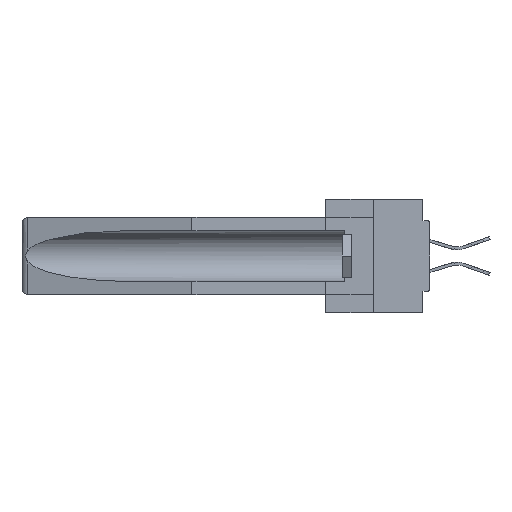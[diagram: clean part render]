
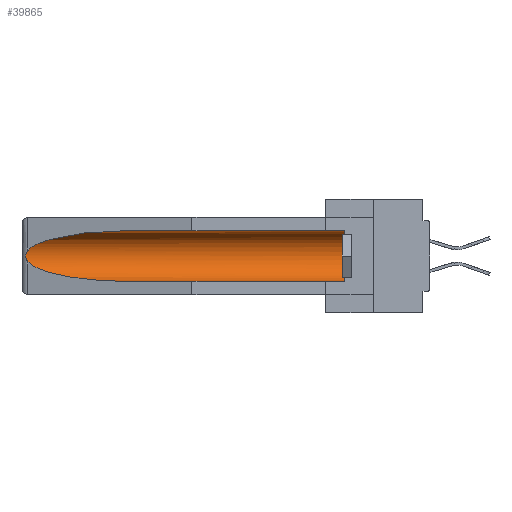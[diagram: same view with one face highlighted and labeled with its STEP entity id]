
A CAD part, left-side view. The second image highlights one B-rep face of the part: STEP entity #39865.
In plain terms, the highlighted cylindrical face has radius 2.857 mm (diameter 5.715 mm), a partial arc.
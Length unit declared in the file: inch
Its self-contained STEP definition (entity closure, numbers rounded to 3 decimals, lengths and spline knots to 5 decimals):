
#250 = B_SPLINE_CURVE_WITH_KNOTS ( 'NONE', 3,
 ( #32908, #36458, #30248, #26725, #6986, #30392, #23396, #7128, #13516, #16598 ),
 .UNSPECIFIED., .F., .F.,
 ( 4, 2, 2, 2, 4 ),
 ( 0., 0.00029, 0.00058, 0.00087, 0.00117 ),
 .UNSPECIFIED. ) ;
#292 = CYLINDRICAL_SURFACE ( 'NONE', #24004, 0.1125 ) ;
#764 = CARTESIAN_POINT ( 'NONE',  ( 0.155, 0.126, -0.284 ) ) ;
#2625 = VECTOR ( 'NONE', #35046, 39.37008 ) ;
#2854 = DIRECTION ( 'NONE',  ( 0., 1., 0. ) ) ;
#3840 = EDGE_CURVE ( 'NONE', #23100, #32858, #10617, .T. ) ;
#4747 = CARTESIAN_POINT ( 'NONE',  ( 0.26537, 1.52718, -0.19328 ) ) ;
#6986 = CARTESIAN_POINT ( 'NONE',  ( 0.2675, 1.53308, -0.16763 ) ) ;
#7058 = CARTESIAN_POINT ( 'NONE',  ( 0.21114, 1.30732, -0.284 ) ) ;
#7128 = CARTESIAN_POINT ( 'NONE',  ( 0.26655, 1.53094, -0.18657 ) ) ;
#7824 = CIRCLE ( 'NONE', #17391, 0.1125 ) ;
#8204 = VECTOR ( 'NONE', #8627, 39.37008 ) ;
#8316 = CARTESIAN_POINT ( 'NONE',  ( 0.155, -0.30754, -0.059 ) ) ;
#8610 = EDGE_CURVE ( 'NONE', #11835, #23100, #250, .T. ) ;
#8627 = DIRECTION ( 'NONE',  ( 0., 1., 0. ) ) ;
#9091 = CARTESIAN_POINT ( 'NONE',  ( 0.21114, 1.30732, -0.059 ) ) ;
#9203 = DIRECTION ( 'NONE',  ( 0., -1., 0. ) ) ;
#10617 =( BOUNDED_CURVE ( )  B_SPLINE_CURVE ( 3, ( #14150, #40654, #7058, #34012 ),
 .UNSPECIFIED., .F., .T. ) 
 B_SPLINE_CURVE_WITH_KNOTS ( ( 4, 4 ),
 ( 0.1948, 1.5708 ),
 .UNSPECIFIED. ) 
 CURVE ( )  GEOMETRIC_REPRESENTATION_ITEM ( )  RATIONAL_B_SPLINE_CURVE ( ( 1., 0.848, 0.848, 1. ) ) 
 REPRESENTATION_ITEM ( '' )  );
#11644 = LINE ( 'NONE', #25319, #2625 ) ;
#11835 = VERTEX_POINT ( 'NONE', #36188 ) ;
#13516 = CARTESIAN_POINT ( 'NONE',  ( 0.26597, 1.5296, -0.19026 ) ) ;
#14150 = CARTESIAN_POINT ( 'NONE',  ( 0.26537, 1.52718, -0.19328 ) ) ;
#15276 = CARTESIAN_POINT ( 'NONE',  ( 0.155, 0.126, -0.059 ) ) ;
#16598 = CARTESIAN_POINT ( 'NONE',  ( 0.26537, 1.52718, -0.19328 ) ) ;
#17274 = ORIENTED_EDGE ( 'NONE', *, *, #36701, .T. ) ;
#17391 = AXIS2_PLACEMENT_3D ( 'NONE', #19543, #9203, #18646 ) ;
#18308 = EDGE_LOOP ( 'NONE', ( #17274, #29156, #29476, #43070, #39761, #18794 ) ) ;
#18436 =( BOUNDED_CURVE ( )  B_SPLINE_CURVE ( 3, ( #19293, #9091, #39552, #19436 ),
 .UNSPECIFIED., .F., .F. ) 
 B_SPLINE_CURVE_WITH_KNOTS ( ( 4, 4 ),
 ( 4.71239, 6.08839 ),
 .UNSPECIFIED. ) 
 CURVE ( )  GEOMETRIC_REPRESENTATION_ITEM ( )  RATIONAL_B_SPLINE_CURVE ( ( 1., 0.848, 0.848, 1. ) ) 
 REPRESENTATION_ITEM ( '' )  );
#18646 = DIRECTION ( 'NONE',  ( 0., 0., 1. ) ) ;
#18794 = ORIENTED_EDGE ( 'NONE', *, *, #40266, .T. ) ;
#19293 = CARTESIAN_POINT ( 'NONE',  ( 0.155, 1.07973, -0.059 ) ) ;
#19436 = CARTESIAN_POINT ( 'NONE',  ( 0.26537, 1.52718, -0.14972 ) ) ;
#19543 = CARTESIAN_POINT ( 'NONE',  ( 0.155, 0.126, -0.1715 ) ) ;
#20162 = EDGE_CURVE ( 'NONE', #38524, #30199, #7824, .T. ) ;
#20185 = CARTESIAN_POINT ( 'NONE',  ( 0.155, -0.30754, -0.1715 ) ) ;
#23100 = VERTEX_POINT ( 'NONE', #4747 ) ;
#23396 = CARTESIAN_POINT ( 'NONE',  ( 0.2673, 1.53269, -0.17917 ) ) ;
#23558 = DIRECTION ( 'NONE',  ( 0., 0., 1. ) ) ;
#24004 = AXIS2_PLACEMENT_3D ( 'NONE', #20185, #2854, #23558 ) ;
#25319 = CARTESIAN_POINT ( 'NONE',  ( 0.155, -0.30754, -0.284 ) ) ;
#26725 = CARTESIAN_POINT ( 'NONE',  ( 0.2673, 1.5327, -0.16383 ) ) ;
#29156 = ORIENTED_EDGE ( 'NONE', *, *, #8610, .T. ) ;
#29476 = ORIENTED_EDGE ( 'NONE', *, *, #3840, .T. ) ;
#30199 = VERTEX_POINT ( 'NONE', #15276 ) ;
#30248 = CARTESIAN_POINT ( 'NONE',  ( 0.26654, 1.53092, -0.15636 ) ) ;
#30392 = CARTESIAN_POINT ( 'NONE',  ( 0.2675, 1.53308, -0.17534 ) ) ;
#32858 = VERTEX_POINT ( 'NONE', #36733 ) ;
#32908 = CARTESIAN_POINT ( 'NONE',  ( 0.26537, 1.52718, -0.14972 ) ) ;
#33502 = LINE ( 'NONE', #8316, #8204 ) ;
#34012 = CARTESIAN_POINT ( 'NONE',  ( 0.155, 1.07973, -0.284 ) ) ;
#34392 = EDGE_CURVE ( 'NONE', #38524, #32858, #11644, .T. ) ;
#35046 = DIRECTION ( 'NONE',  ( 0., 1., 0. ) ) ;
#35195 = VERTEX_POINT ( 'NONE', #40995 ) ;
#36188 = CARTESIAN_POINT ( 'NONE',  ( 0.26537, 1.52718, -0.14972 ) ) ;
#36458 = CARTESIAN_POINT ( 'NONE',  ( 0.26597, 1.52961, -0.15275 ) ) ;
#36701 = EDGE_CURVE ( 'NONE', #35195, #11835, #18436, .T. ) ;
#36733 = CARTESIAN_POINT ( 'NONE',  ( 0.155, 1.07973, -0.284 ) ) ;
#38524 = VERTEX_POINT ( 'NONE', #764 ) ;
#39552 = CARTESIAN_POINT ( 'NONE',  ( 0.25451, 1.48313, -0.09465 ) ) ;
#39761 = ORIENTED_EDGE ( 'NONE', *, *, #20162, .T. ) ;
#39865 = ADVANCED_FACE ( 'NONE', ( #41485 ), #292, .F. ) ;
#40266 = EDGE_CURVE ( 'NONE', #30199, #35195, #33502, .T. ) ;
#40654 = CARTESIAN_POINT ( 'NONE',  ( 0.25451, 1.48313, -0.24835 ) ) ;
#40995 = CARTESIAN_POINT ( 'NONE',  ( 0.155, 1.07973, -0.059 ) ) ;
#41485 = FACE_OUTER_BOUND ( 'NONE', #18308, .T. ) ;
#43070 = ORIENTED_EDGE ( 'NONE', *, *, #34392, .F. ) ;
